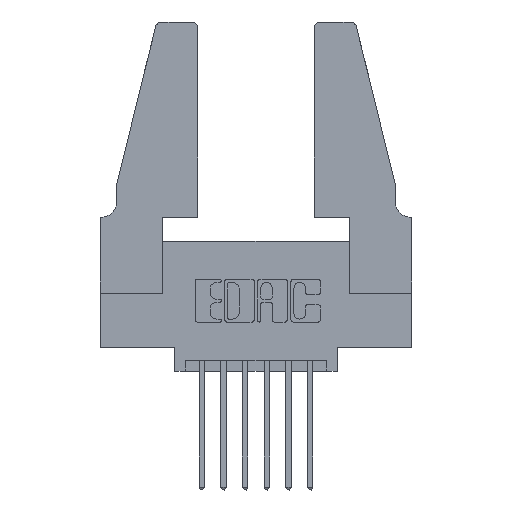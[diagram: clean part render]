
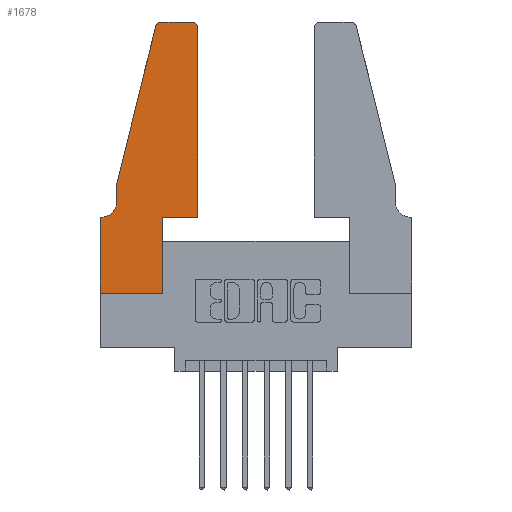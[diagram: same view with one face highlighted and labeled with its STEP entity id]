
A CAD part, top view. The second image highlights one B-rep face of the part: STEP entity #1678.
In plain terms, the highlighted planar face has unit normal (0, 0, 1).
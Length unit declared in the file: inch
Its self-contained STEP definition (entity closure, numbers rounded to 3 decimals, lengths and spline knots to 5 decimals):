
#10 = LINE ( 'NONE', #5795, #1977 ) ;
#68 = CIRCLE ( 'NONE', #1405, 0.03 ) ;
#153 = DIRECTION ( 'NONE',  ( 1., 0., 0. ) ) ;
#197 = DIRECTION ( 'NONE',  ( -1., 0., 0. ) ) ;
#419 = ORIENTED_EDGE ( 'NONE', *, *, #7980, .T. ) ;
#722 = CARTESIAN_POINT ( 'NONE',  ( 0.4505, 0.35, 0.37 ) ) ;
#893 = VERTEX_POINT ( 'NONE', #6463 ) ;
#1002 = VERTEX_POINT ( 'NONE', #1870 ) ;
#1094 = CARTESIAN_POINT ( 'NONE',  ( 0.4205, 1.25, 0.37 ) ) ;
#1157 = ORIENTED_EDGE ( 'NONE', *, *, #7563, .T. ) ;
#1304 = FACE_OUTER_BOUND ( 'NONE', #7125, .T. ) ;
#1331 = VERTEX_POINT ( 'NONE', #6238 ) ;
#1405 = AXIS2_PLACEMENT_3D ( 'NONE', #3316, #3140, #3091 ) ;
#1622 = CARTESIAN_POINT ( 'NONE',  ( 0.0755, 0.5, 0.37 ) ) ;
#1678 = ADVANCED_FACE ( 'NONE', ( #1304 ), #6245, .T. ) ;
#1680 = ORIENTED_EDGE ( 'NONE', *, *, #5497, .T. ) ;
#1769 = DIRECTION ( 'NONE',  ( -1., 0., 0. ) ) ;
#1870 = CARTESIAN_POINT ( 'NONE',  ( 0.4505, 1.22, 0.37 ) ) ;
#1977 = VECTOR ( 'NONE', #6004, 39.37008 ) ;
#2004 = ORIENTED_EDGE ( 'NONE', *, *, #3250, .T. ) ;
#2072 = ORIENTED_EDGE ( 'NONE', *, *, #11504, .T. ) ;
#2109 = VERTEX_POINT ( 'NONE', #10677 ) ;
#2171 = VERTEX_POINT ( 'NONE', #2245 ) ;
#2245 = CARTESIAN_POINT ( 'NONE',  ( 0.284, 1.25, 0.37 ) ) ;
#2582 = LINE ( 'NONE', #4620, #7442 ) ;
#2604 = ORIENTED_EDGE ( 'NONE', *, *, #11622, .T. ) ;
#2606 = DIRECTION ( 'NONE',  ( 0., 1., 0. ) ) ;
#2638 = VERTEX_POINT ( 'NONE', #1622 ) ;
#2672 = CIRCLE ( 'NONE', #10193, 0.07 ) ;
#3091 = DIRECTION ( 'NONE',  ( 1., 0., 0. ) ) ;
#3140 = DIRECTION ( 'NONE',  ( 0., 0., 1. ) ) ;
#3200 = CARTESIAN_POINT ( 'NONE',  ( 0., 0., 0.37 ) ) ;
#3250 = EDGE_CURVE ( 'NONE', #2171, #893, #68, .T. ) ;
#3316 = CARTESIAN_POINT ( 'NONE',  ( 0.284, 1.22, 0.37 ) ) ;
#3324 = CARTESIAN_POINT ( 'NONE',  ( 0.2865, 0., 0.37 ) ) ;
#3337 = VERTEX_POINT ( 'NONE', #3324 ) ;
#3470 = ORIENTED_EDGE ( 'NONE', *, *, #4315, .T. ) ;
#3474 = CARTESIAN_POINT ( 'NONE',  ( 0.4205, 1.22, 0.37 ) ) ;
#3682 = CARTESIAN_POINT ( 'NONE',  ( 0.0755, 0.42, 0.37 ) ) ;
#3858 = VECTOR ( 'NONE', #6271, 39.37008 ) ;
#3916 = VERTEX_POINT ( 'NONE', #3200 ) ;
#3936 = CARTESIAN_POINT ( 'NONE',  ( 0., 0., 0.37 ) ) ;
#4142 = CIRCLE ( 'NONE', #9470, 0.03 ) ;
#4315 = EDGE_CURVE ( 'NONE', #893, #2638, #4926, .T. ) ;
#4388 = DIRECTION ( 'NONE',  ( 1., 0., 0. ) ) ;
#4482 = VECTOR ( 'NONE', #197, 39.37008 ) ;
#4620 = CARTESIAN_POINT ( 'NONE',  ( 0., 0., 0.37 ) ) ;
#4844 = ORIENTED_EDGE ( 'NONE', *, *, #8399, .T. ) ;
#4908 = CARTESIAN_POINT ( 'NONE',  ( 0.0755, 0.35, 0.37 ) ) ;
#4926 = LINE ( 'NONE', #7778, #8170 ) ;
#4995 = LINE ( 'NONE', #3936, #9480 ) ;
#5180 = DIRECTION ( 'NONE',  ( 0., 0., -1. ) ) ;
#5497 = EDGE_CURVE ( 'NONE', #2638, #9598, #10, .T. ) ;
#5566 = DIRECTION ( 'NONE',  ( 0., -1., 0. ) ) ;
#5633 = CARTESIAN_POINT ( 'NONE',  ( 0.2605, 1.25, 0.37 ) ) ;
#5795 = CARTESIAN_POINT ( 'NONE',  ( 0.0755, 0.5, 0.37 ) ) ;
#6004 = DIRECTION ( 'NONE',  ( 0., -1., 0. ) ) ;
#6163 = VECTOR ( 'NONE', #1769, 39.37008 ) ;
#6238 = CARTESIAN_POINT ( 'NONE',  ( 0.4505, 0.35, 0.37 ) ) ;
#6245 = PLANE ( 'NONE',  #6346 ) ;
#6271 = DIRECTION ( 'NONE',  ( 1., 0., 0. ) ) ;
#6346 = AXIS2_PLACEMENT_3D ( 'NONE', #10377, #10404, #10392 ) ;
#6463 = CARTESIAN_POINT ( 'NONE',  ( 0.25487, 1.22718, 0.37 ) ) ;
#6640 = VERTEX_POINT ( 'NONE', #8026 ) ;
#6921 = LINE ( 'NONE', #4908, #4482 ) ;
#6928 = CARTESIAN_POINT ( 'NONE',  ( 0.4505, 0.35, 0.37 ) ) ;
#6975 = EDGE_CURVE ( 'NONE', #11639, #1331, #8664, .T. ) ;
#7005 = CARTESIAN_POINT ( 'NONE',  ( 0.2865, 0.35, 0.37 ) ) ;
#7125 = EDGE_LOOP ( 'NONE', ( #2604, #2004, #3470, #1680, #7798, #419, #4844, #11741, #2072, #9062, #10902, #1157 ) ) ;
#7243 = VERTEX_POINT ( 'NONE', #1094 ) ;
#7405 = CARTESIAN_POINT ( 'NONE',  ( 0.2865, 0.35, 0.37 ) ) ;
#7442 = VECTOR ( 'NONE', #5566, 39.37008 ) ;
#7563 = EDGE_CURVE ( 'NONE', #1002, #7243, #4142, .T. ) ;
#7775 = DIRECTION ( 'NONE',  ( -0.239, -0.971, 0. ) ) ;
#7778 = CARTESIAN_POINT ( 'NONE',  ( 0.0755, 0.5, 0.37 ) ) ;
#7798 = ORIENTED_EDGE ( 'NONE', *, *, #11486, .T. ) ;
#7980 = EDGE_CURVE ( 'NONE', #6640, #2109, #6921, .T. ) ;
#8026 = CARTESIAN_POINT ( 'NONE',  ( 0.0055, 0.35, 0.37 ) ) ;
#8170 = VECTOR ( 'NONE', #7775, 39.37008 ) ;
#8399 = EDGE_CURVE ( 'NONE', #2109, #3916, #2582, .T. ) ;
#8504 = LINE ( 'NONE', #5633, #6163 ) ;
#8664 = LINE ( 'NONE', #6928, #3858 ) ;
#8819 = VECTOR ( 'NONE', #2606, 39.37008 ) ;
#9062 = ORIENTED_EDGE ( 'NONE', *, *, #6975, .T. ) ;
#9322 = VECTOR ( 'NONE', #10527, 39.37008 ) ;
#9470 = AXIS2_PLACEMENT_3D ( 'NONE', #3474, #9787, #4388 ) ;
#9480 = VECTOR ( 'NONE', #153, 39.37008 ) ;
#9518 = EDGE_CURVE ( 'NONE', #1331, #1002, #11770, .T. ) ;
#9598 = VERTEX_POINT ( 'NONE', #3682 ) ;
#9628 = LINE ( 'NONE', #7005, #9322 ) ;
#9787 = DIRECTION ( 'NONE',  ( 0., 0., 1. ) ) ;
#10193 = AXIS2_PLACEMENT_3D ( 'NONE', #10562, #5180, #11446 ) ;
#10377 = CARTESIAN_POINT ( 'NONE',  ( 0., 0.35, 0.37 ) ) ;
#10392 = DIRECTION ( 'NONE',  ( 1., 0., 0. ) ) ;
#10404 = DIRECTION ( 'NONE',  ( 0., 0., 1. ) ) ;
#10527 = DIRECTION ( 'NONE',  ( 0., 1., 0. ) ) ;
#10562 = CARTESIAN_POINT ( 'NONE',  ( 0.0055, 0.42, 0.37 ) ) ;
#10605 = EDGE_CURVE ( 'NONE', #3916, #3337, #4995, .T. ) ;
#10677 = CARTESIAN_POINT ( 'NONE',  ( 0., 0.35, 0.37 ) ) ;
#10902 = ORIENTED_EDGE ( 'NONE', *, *, #9518, .T. ) ;
#11446 = DIRECTION ( 'NONE',  ( -1., 0., 0. ) ) ;
#11486 = EDGE_CURVE ( 'NONE', #9598, #6640, #2672, .T. ) ;
#11504 = EDGE_CURVE ( 'NONE', #3337, #11639, #9628, .T. ) ;
#11622 = EDGE_CURVE ( 'NONE', #7243, #2171, #8504, .T. ) ;
#11639 = VERTEX_POINT ( 'NONE', #7405 ) ;
#11741 = ORIENTED_EDGE ( 'NONE', *, *, #10605, .T. ) ;
#11770 = LINE ( 'NONE', #722, #8819 ) ;
